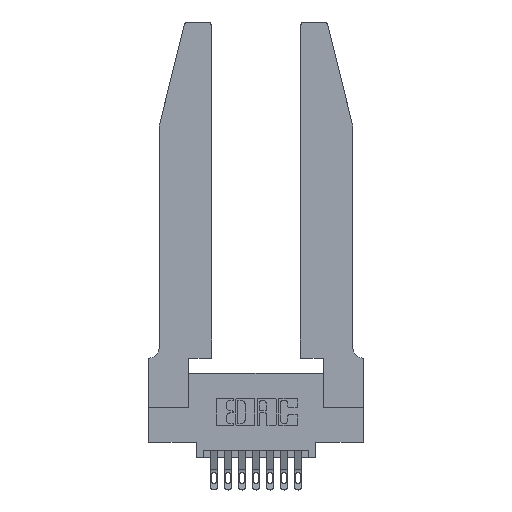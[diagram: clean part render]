
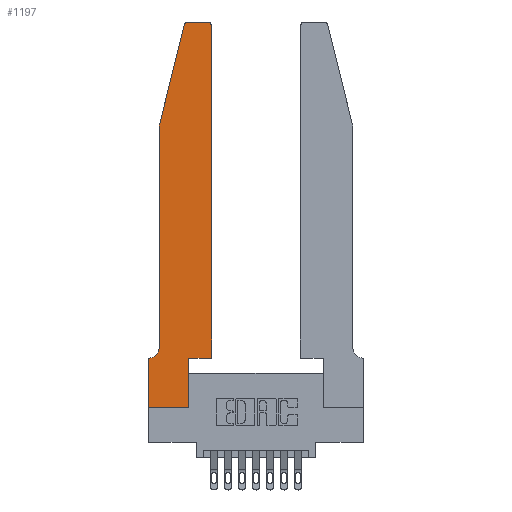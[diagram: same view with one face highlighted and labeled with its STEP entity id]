
A CAD part, top view. The second image highlights one B-rep face of the part: STEP entity #1197.
In plain terms, the highlighted planar face has unit normal (0, 0, 1).
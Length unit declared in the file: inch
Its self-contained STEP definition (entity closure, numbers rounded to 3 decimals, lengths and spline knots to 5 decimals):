
#544 = CARTESIAN_POINT ( 'NONE',  ( 0.0755, 2., 0.37 ) ) ;
#670 = ORIENTED_EDGE ( 'NONE', *, *, #7311, .T. ) ;
#855 = VECTOR ( 'NONE', #8247, 39.37008 ) ;
#869 = EDGE_CURVE ( 'NONE', #5811, #1459, #10135, .T. ) ;
#894 = CARTESIAN_POINT ( 'NONE',  ( 0.4205, 2.75, 0.37 ) ) ;
#977 = DIRECTION ( 'NONE',  ( -1., 0., 0. ) ) ;
#1085 = DIRECTION ( 'NONE',  ( -1., 0., 0. ) ) ;
#1147 = DIRECTION ( 'NONE',  ( 1., 0., 0. ) ) ;
#1197 = ADVANCED_FACE ( 'NONE', ( #6825 ), #5079, .T. ) ;
#1224 = CARTESIAN_POINT ( 'NONE',  ( 0.0755, 2., 0.37 ) ) ;
#1357 = CARTESIAN_POINT ( 'NONE',  ( 0., 0., 0.37 ) ) ;
#1459 = VERTEX_POINT ( 'NONE', #544 ) ;
#1629 = CARTESIAN_POINT ( 'NONE',  ( 0.2605, 2.75, 0.37 ) ) ;
#1643 = VECTOR ( 'NONE', #10482, 39.37008 ) ;
#1808 = VERTEX_POINT ( 'NONE', #13790 ) ;
#1844 = EDGE_CURVE ( 'NONE', #1808, #13812, #14224, .T. ) ;
#2128 = AXIS2_PLACEMENT_3D ( 'NONE', #15325, #8468, #1147 ) ;
#2455 = ORIENTED_EDGE ( 'NONE', *, *, #1844, .T. ) ;
#2783 = EDGE_LOOP ( 'NONE', ( #11632, #8158, #10122, #13685, #12604, #7027, #2455, #5066, #670, #12548, #7148, #8984 ) ) ;
#2884 = VERTEX_POINT ( 'NONE', #14910 ) ;
#2946 = EDGE_CURVE ( 'NONE', #7356, #1808, #15276, .T. ) ;
#3067 = DIRECTION ( 'NONE',  ( 0., 1., 0. ) ) ;
#3687 = DIRECTION ( 'NONE',  ( 1., 0., 0. ) ) ;
#3874 = AXIS2_PLACEMENT_3D ( 'NONE', #15085, #11849, #9815 ) ;
#3938 = VERTEX_POINT ( 'NONE', #9093 ) ;
#4069 = EDGE_CURVE ( 'NONE', #3938, #8060, #8058, .T. ) ;
#4679 = CARTESIAN_POINT ( 'NONE',  ( 0.4205, 2.72, 0.37 ) ) ;
#4957 = CARTESIAN_POINT ( 'NONE',  ( 0.4505, 0.35, 0.37 ) ) ;
#5066 = ORIENTED_EDGE ( 'NONE', *, *, #10330, .T. ) ;
#5079 = PLANE ( 'NONE',  #3874 ) ;
#5456 = EDGE_CURVE ( 'NONE', #14207, #8698, #9476, .T. ) ;
#5811 = VERTEX_POINT ( 'NONE', #10938 ) ;
#5887 = DIRECTION ( 'NONE',  ( 1., 0., 0. ) ) ;
#6124 = CARTESIAN_POINT ( 'NONE',  ( 0., 0., 0.37 ) ) ;
#6146 = LINE ( 'NONE', #6124, #8208 ) ;
#6611 = LINE ( 'NONE', #4957, #9766 ) ;
#6825 = FACE_OUTER_BOUND ( 'NONE', #2783, .T. ) ;
#7027 = ORIENTED_EDGE ( 'NONE', *, *, #2946, .T. ) ;
#7148 = ORIENTED_EDGE ( 'NONE', *, *, #4069, .T. ) ;
#7311 = EDGE_CURVE ( 'NONE', #2884, #15168, #11768, .T. ) ;
#7356 = VERTEX_POINT ( 'NONE', #14912 ) ;
#7383 = CIRCLE ( 'NONE', #10327, 0.03 ) ;
#7531 = EDGE_CURVE ( 'NONE', #9840, #7356, #11945, .T. ) ;
#8058 = LINE ( 'NONE', #8334, #13422 ) ;
#8060 = VERTEX_POINT ( 'NONE', #10796 ) ;
#8113 = VECTOR ( 'NONE', #11740, 39.37008 ) ;
#8158 = ORIENTED_EDGE ( 'NONE', *, *, #13676, .T. ) ;
#8208 = VECTOR ( 'NONE', #3687, 39.37008 ) ;
#8247 = DIRECTION ( 'NONE',  ( -0.239, -0.971, 0. ) ) ;
#8334 = CARTESIAN_POINT ( 'NONE',  ( 0.4505, 0.35, 0.37 ) ) ;
#8405 = DIRECTION ( 'NONE',  ( 0., 0., -1. ) ) ;
#8468 = DIRECTION ( 'NONE',  ( 0., 0., 1. ) ) ;
#8698 = VERTEX_POINT ( 'NONE', #9921 ) ;
#8720 = VECTOR ( 'NONE', #3067, 39.37008 ) ;
#8984 = ORIENTED_EDGE ( 'NONE', *, *, #9103, .T. ) ;
#9053 = EDGE_CURVE ( 'NONE', #1459, #9840, #11170, .T. ) ;
#9093 = CARTESIAN_POINT ( 'NONE',  ( 0.4505, 0.35, 0.37 ) ) ;
#9103 = EDGE_CURVE ( 'NONE', #8060, #14207, #7383, .T. ) ;
#9189 = EDGE_CURVE ( 'NONE', #15168, #3938, #6611, .T. ) ;
#9335 = CARTESIAN_POINT ( 'NONE',  ( 0.0755, 2., 0.37 ) ) ;
#9476 = LINE ( 'NONE', #1629, #12152 ) ;
#9677 = CARTESIAN_POINT ( 'NONE',  ( 0.0755, 0.42, 0.37 ) ) ;
#9766 = VECTOR ( 'NONE', #12022, 39.37008 ) ;
#9815 = DIRECTION ( 'NONE',  ( 1., 0., 0. ) ) ;
#9840 = VERTEX_POINT ( 'NONE', #9677 ) ;
#9921 = CARTESIAN_POINT ( 'NONE',  ( 0.284, 2.75, 0.37 ) ) ;
#10063 = DIRECTION ( 'NONE',  ( -1., 0., 0. ) ) ;
#10122 = ORIENTED_EDGE ( 'NONE', *, *, #869, .T. ) ;
#10135 = LINE ( 'NONE', #1224, #855 ) ;
#10226 = CARTESIAN_POINT ( 'NONE',  ( 0.2865, 0.35, 0.37 ) ) ;
#10327 = AXIS2_PLACEMENT_3D ( 'NONE', #4679, #12853, #5887 ) ;
#10330 = EDGE_CURVE ( 'NONE', #13812, #2884, #6146, .T. ) ;
#10482 = DIRECTION ( 'NONE',  ( 0., -1., 0. ) ) ;
#10598 = DIRECTION ( 'NONE',  ( 0., 1., 0. ) ) ;
#10796 = CARTESIAN_POINT ( 'NONE',  ( 0.4505, 2.72, 0.37 ) ) ;
#10938 = CARTESIAN_POINT ( 'NONE',  ( 0.25487, 2.72718, 0.37 ) ) ;
#11170 = LINE ( 'NONE', #9335, #1643 ) ;
#11632 = ORIENTED_EDGE ( 'NONE', *, *, #5456, .T. ) ;
#11740 = DIRECTION ( 'NONE',  ( 0., -1., 0. ) ) ;
#11767 = CARTESIAN_POINT ( 'NONE',  ( 0.0755, 0.35, 0.37 ) ) ;
#11768 = LINE ( 'NONE', #12440, #8720 ) ;
#11849 = DIRECTION ( 'NONE',  ( 0., 0., 1. ) ) ;
#11945 = CIRCLE ( 'NONE', #14046, 0.07 ) ;
#12022 = DIRECTION ( 'NONE',  ( 1., 0., 0. ) ) ;
#12152 = VECTOR ( 'NONE', #10063, 39.37008 ) ;
#12440 = CARTESIAN_POINT ( 'NONE',  ( 0.2865, 0.35, 0.37 ) ) ;
#12548 = ORIENTED_EDGE ( 'NONE', *, *, #9189, .T. ) ;
#12551 = VECTOR ( 'NONE', #977, 39.37008 ) ;
#12604 = ORIENTED_EDGE ( 'NONE', *, *, #7531, .T. ) ;
#12853 = DIRECTION ( 'NONE',  ( 0., 0., 1. ) ) ;
#13304 = CARTESIAN_POINT ( 'NONE',  ( 0., 0., 0.37 ) ) ;
#13422 = VECTOR ( 'NONE', #10598, 39.37008 ) ;
#13676 = EDGE_CURVE ( 'NONE', #8698, #5811, #13820, .T. ) ;
#13685 = ORIENTED_EDGE ( 'NONE', *, *, #9053, .T. ) ;
#13790 = CARTESIAN_POINT ( 'NONE',  ( 0., 0.35, 0.37 ) ) ;
#13812 = VERTEX_POINT ( 'NONE', #1357 ) ;
#13820 = CIRCLE ( 'NONE', #2128, 0.03 ) ;
#14046 = AXIS2_PLACEMENT_3D ( 'NONE', #15262, #8405, #1085 ) ;
#14207 = VERTEX_POINT ( 'NONE', #894 ) ;
#14224 = LINE ( 'NONE', #13304, #8113 ) ;
#14910 = CARTESIAN_POINT ( 'NONE',  ( 0.2865, 0., 0.37 ) ) ;
#14912 = CARTESIAN_POINT ( 'NONE',  ( 0.0055, 0.35, 0.37 ) ) ;
#15085 = CARTESIAN_POINT ( 'NONE',  ( 0., 0.35, 0.37 ) ) ;
#15168 = VERTEX_POINT ( 'NONE', #10226 ) ;
#15262 = CARTESIAN_POINT ( 'NONE',  ( 0.0055, 0.42, 0.37 ) ) ;
#15276 = LINE ( 'NONE', #11767, #12551 ) ;
#15325 = CARTESIAN_POINT ( 'NONE',  ( 0.284, 2.72, 0.37 ) ) ;
